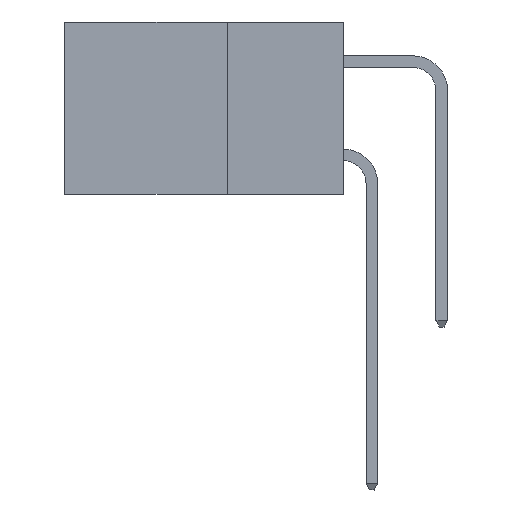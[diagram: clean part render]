
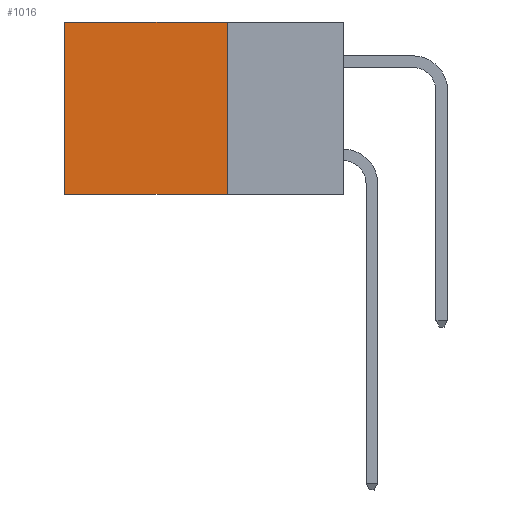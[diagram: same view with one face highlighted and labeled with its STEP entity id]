
A CAD part, left-side view. The second image highlights one B-rep face of the part: STEP entity #1016.
In plain terms, the highlighted planar face has unit normal (-1, 0, 0).
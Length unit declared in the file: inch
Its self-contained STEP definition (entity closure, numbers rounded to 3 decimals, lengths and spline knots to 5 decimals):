
#1016 = ADVANCED_FACE ( 'NONE', ( #16733 ), #17443, .F. ) ;
#1773 = ORIENTED_EDGE ( 'NONE', *, *, #17400, .F. ) ;
#2384 = DIRECTION ( 'NONE',  ( 0., 1., 0. ) ) ;
#4398 = LINE ( 'NONE', #19250, #25907 ) ;
#4585 = DIRECTION ( 'NONE',  ( 0., 0., -1. ) ) ;
#4769 = AXIS2_PLACEMENT_3D ( 'NONE', #17421, #5385, #4585 ) ;
#5054 = CARTESIAN_POINT ( 'NONE',  ( 0.298, 0.25, -0.37 ) ) ;
#5140 = EDGE_CURVE ( 'NONE', #20192, #23217, #8666, .T. ) ;
#5385 = DIRECTION ( 'NONE',  ( 1., 0., 0. ) ) ;
#6759 = ORIENTED_EDGE ( 'NONE', *, *, #5140, .T. ) ;
#8142 = VECTOR ( 'NONE', #18427, 39.37008 ) ;
#8471 = ORIENTED_EDGE ( 'NONE', *, *, #15725, .T. ) ;
#8666 = LINE ( 'NONE', #8764, #14252 ) ;
#8764 = CARTESIAN_POINT ( 'NONE',  ( 0.298, 0.25, 0. ) ) ;
#10008 = VECTOR ( 'NONE', #13454, 39.37008 ) ;
#10895 = DIRECTION ( 'NONE',  ( 0., 0., -1. ) ) ;
#11331 = CARTESIAN_POINT ( 'NONE',  ( 0.298, 0.25, 0. ) ) ;
#13454 = DIRECTION ( 'NONE',  ( 0., 1., 0. ) ) ;
#14104 = CARTESIAN_POINT ( 'NONE',  ( 0.298, 0.6, -0.37 ) ) ;
#14252 = VECTOR ( 'NONE', #2384, 39.37008 ) ;
#14272 = CARTESIAN_POINT ( 'NONE',  ( 0.298, 0.6, 0. ) ) ;
#15725 = EDGE_CURVE ( 'NONE', #23217, #16976, #25967, .T. ) ;
#16733 = FACE_OUTER_BOUND ( 'NONE', #17961, .T. ) ;
#16976 = VERTEX_POINT ( 'NONE', #14104 ) ;
#17400 = EDGE_CURVE ( 'NONE', #19351, #16976, #27145, .T. ) ;
#17421 = CARTESIAN_POINT ( 'NONE',  ( 0.298, 0.25, 0. ) ) ;
#17443 = PLANE ( 'NONE',  #4769 ) ;
#17961 = EDGE_LOOP ( 'NONE', ( #8471, #1773, #24980, #6759 ) ) ;
#18427 = DIRECTION ( 'NONE',  ( 0., 0., -1. ) ) ;
#19250 = CARTESIAN_POINT ( 'NONE',  ( 0.298, 0.25, 0. ) ) ;
#19351 = VERTEX_POINT ( 'NONE', #5054 ) ;
#19676 = CARTESIAN_POINT ( 'NONE',  ( 0.298, 0.25, -0.37 ) ) ;
#20192 = VERTEX_POINT ( 'NONE', #11331 ) ;
#23217 = VERTEX_POINT ( 'NONE', #25375 ) ;
#24980 = ORIENTED_EDGE ( 'NONE', *, *, #25874, .F. ) ;
#25375 = CARTESIAN_POINT ( 'NONE',  ( 0.298, 0.6, 0. ) ) ;
#25874 = EDGE_CURVE ( 'NONE', #20192, #19351, #4398, .T. ) ;
#25907 = VECTOR ( 'NONE', #10895, 39.37008 ) ;
#25967 = LINE ( 'NONE', #14272, #8142 ) ;
#27145 = LINE ( 'NONE', #19676, #10008 ) ;
